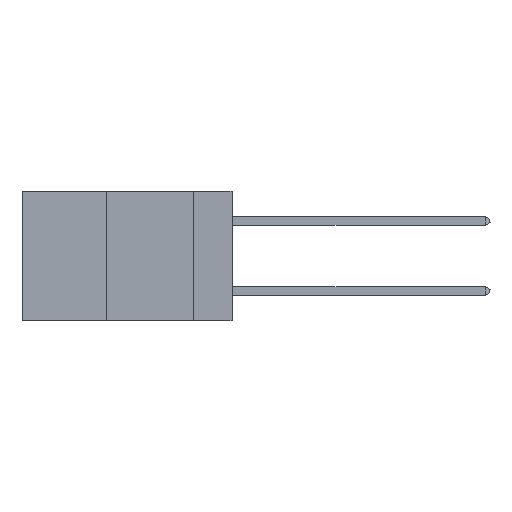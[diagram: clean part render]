
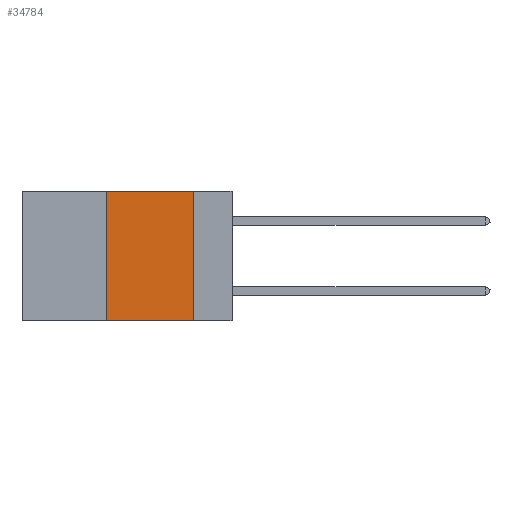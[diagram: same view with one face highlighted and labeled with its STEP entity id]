
A CAD part, left-side view. The second image highlights one B-rep face of the part: STEP entity #34784.
In plain terms, the highlighted planar face has unit normal (-1, 0, 0).
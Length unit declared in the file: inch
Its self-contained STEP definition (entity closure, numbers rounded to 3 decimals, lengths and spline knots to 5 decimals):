
#1159 = EDGE_CURVE ( 'NONE', #11394, #38888, #20214, .T. ) ;
#2375 = DIRECTION ( 'NONE',  ( 0., -1., 0. ) ) ;
#3867 = LINE ( 'NONE', #36213, #4365 ) ;
#4365 = VECTOR ( 'NONE', #2375, 39.37008 ) ;
#6090 = VERTEX_POINT ( 'NONE', #16296 ) ;
#6784 = EDGE_CURVE ( 'NONE', #12992, #6090, #34231, .T. ) ;
#7582 = ORIENTED_EDGE ( 'NONE', *, *, #6784, .F. ) ;
#7678 = ORIENTED_EDGE ( 'NONE', *, *, #15150, .T. ) ;
#8595 = EDGE_LOOP ( 'NONE', ( #7582, #20964, #24752, #7678 ) ) ;
#10383 = CARTESIAN_POINT ( 'NONE',  ( 0., 0.6, -0.37 ) ) ;
#10638 = LINE ( 'NONE', #10383, #16813 ) ;
#11394 = VERTEX_POINT ( 'NONE', #30903 ) ;
#11625 = VECTOR ( 'NONE', #37883, 39.37008 ) ;
#11866 = AXIS2_PLACEMENT_3D ( 'NONE', #16787, #13835, #14106 ) ;
#12992 = VERTEX_POINT ( 'NONE', #17912 ) ;
#13179 = CARTESIAN_POINT ( 'NONE',  ( 0., 0.11, 0. ) ) ;
#13446 = DIRECTION ( 'NONE',  ( 0., 0., -1. ) ) ;
#13835 = DIRECTION ( 'NONE',  ( 1., 0., 0. ) ) ;
#14106 = DIRECTION ( 'NONE',  ( 0., 0., -1. ) ) ;
#15150 = EDGE_CURVE ( 'NONE', #11394, #6090, #10638, .T. ) ;
#16296 = CARTESIAN_POINT ( 'NONE',  ( 0., 0.11, -0.37 ) ) ;
#16787 = CARTESIAN_POINT ( 'NONE',  ( 0., 0.6, 0. ) ) ;
#16813 = VECTOR ( 'NONE', #24989, 39.37008 ) ;
#17912 = CARTESIAN_POINT ( 'NONE',  ( 0., 0.11, 0. ) ) ;
#20214 = LINE ( 'NONE', #34820, #11625 ) ;
#20964 = ORIENTED_EDGE ( 'NONE', *, *, #33672, .F. ) ;
#23022 = PLANE ( 'NONE',  #11866 ) ;
#24752 = ORIENTED_EDGE ( 'NONE', *, *, #1159, .F. ) ;
#24989 = DIRECTION ( 'NONE',  ( 0., -1., 0. ) ) ;
#29419 = FACE_OUTER_BOUND ( 'NONE', #8595, .T. ) ;
#30903 = CARTESIAN_POINT ( 'NONE',  ( 0., 0.36, -0.37 ) ) ;
#33672 = EDGE_CURVE ( 'NONE', #38888, #12992, #3867, .T. ) ;
#34231 = LINE ( 'NONE', #13179, #34699 ) ;
#34256 = CARTESIAN_POINT ( 'NONE',  ( 0., 0.36, 0. ) ) ;
#34699 = VECTOR ( 'NONE', #13446, 39.37008 ) ;
#34784 = ADVANCED_FACE ( 'NONE', ( #29419 ), #23022, .F. ) ;
#34820 = CARTESIAN_POINT ( 'NONE',  ( 0., 0.36, 0. ) ) ;
#36213 = CARTESIAN_POINT ( 'NONE',  ( 0., 0.6, 0. ) ) ;
#37883 = DIRECTION ( 'NONE',  ( 0., 0., 1. ) ) ;
#38888 = VERTEX_POINT ( 'NONE', #34256 ) ;
